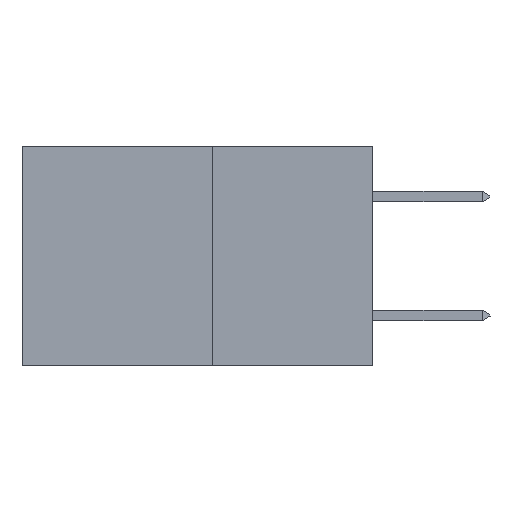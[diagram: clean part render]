
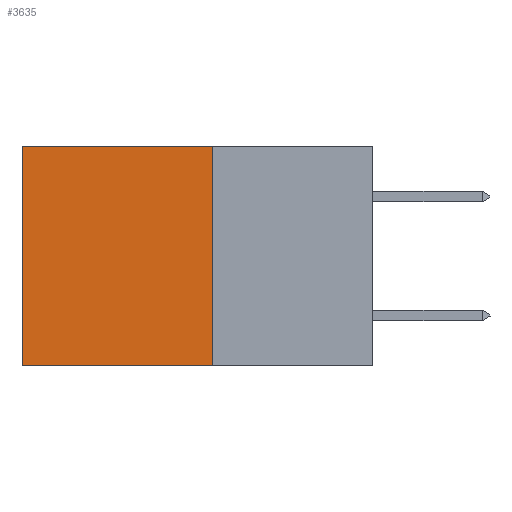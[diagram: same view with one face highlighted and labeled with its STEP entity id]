
A CAD part, left-side view. The second image highlights one B-rep face of the part: STEP entity #3635.
In plain terms, the highlighted planar face has unit normal (-1, 0, 0).
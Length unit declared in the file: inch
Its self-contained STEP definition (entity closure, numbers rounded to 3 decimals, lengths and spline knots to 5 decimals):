
#110 = VECTOR ( 'NONE', #1015, 39.37008 ) ;
#155 = CARTESIAN_POINT ( 'NONE',  ( 0.277, 0.27, -0.37 ) ) ;
#812 = CARTESIAN_POINT ( 'NONE',  ( 0.277, 0.59, -0.37 ) ) ;
#900 = ORIENTED_EDGE ( 'NONE', *, *, #6768, .F. ) ;
#988 = VECTOR ( 'NONE', #1818, 39.37008 ) ;
#1015 = DIRECTION ( 'NONE',  ( 0., 1., 0. ) ) ;
#1137 = DIRECTION ( 'NONE',  ( 1., 0., 0. ) ) ;
#1166 = DIRECTION ( 'NONE',  ( 0., 0., -1. ) ) ;
#1189 = PLANE ( 'NONE',  #7337 ) ;
#1203 = CARTESIAN_POINT ( 'NONE',  ( 0.277, 0.27, -0.37 ) ) ;
#1358 = EDGE_CURVE ( 'NONE', #4739, #5498, #2336, .T. ) ;
#1521 = EDGE_CURVE ( 'NONE', #5498, #5710, #2466, .T. ) ;
#1818 = DIRECTION ( 'NONE',  ( 0., 0., -1. ) ) ;
#1840 = DIRECTION ( 'NONE',  ( 0., 0., -1. ) ) ;
#1923 = ORIENTED_EDGE ( 'NONE', *, *, #1358, .T. ) ;
#2117 = FACE_OUTER_BOUND ( 'NONE', #4970, .T. ) ;
#2203 = VECTOR ( 'NONE', #1840, 39.37008 ) ;
#2336 = LINE ( 'NONE', #2471, #110 ) ;
#2352 = CARTESIAN_POINT ( 'NONE',  ( 0.277, 0.59, 0. ) ) ;
#2466 = LINE ( 'NONE', #812, #2203 ) ;
#2471 = CARTESIAN_POINT ( 'NONE',  ( 0.277, 0.27, 0. ) ) ;
#2958 = LINE ( 'NONE', #155, #988 ) ;
#3508 = VERTEX_POINT ( 'NONE', #5075 ) ;
#3635 = ADVANCED_FACE ( 'NONE', ( #2117 ), #1189, .F. ) ;
#3849 = DIRECTION ( 'NONE',  ( 0., 1., 0. ) ) ;
#4739 = VERTEX_POINT ( 'NONE', #9595 ) ;
#4970 = EDGE_LOOP ( 'NONE', ( #8831, #900, #5209, #1923 ) ) ;
#5075 = CARTESIAN_POINT ( 'NONE',  ( 0.277, 0.27, -0.37 ) ) ;
#5209 = ORIENTED_EDGE ( 'NONE', *, *, #7965, .F. ) ;
#5498 = VERTEX_POINT ( 'NONE', #2352 ) ;
#5710 = VERTEX_POINT ( 'NONE', #6478 ) ;
#6478 = CARTESIAN_POINT ( 'NONE',  ( 0.277, 0.59, -0.37 ) ) ;
#6768 = EDGE_CURVE ( 'NONE', #3508, #5710, #7169, .T. ) ;
#6955 = VECTOR ( 'NONE', #3849, 39.37008 ) ;
#7169 = LINE ( 'NONE', #9732, #6955 ) ;
#7337 = AXIS2_PLACEMENT_3D ( 'NONE', #1203, #1137, #1166 ) ;
#7965 = EDGE_CURVE ( 'NONE', #4739, #3508, #2958, .T. ) ;
#8831 = ORIENTED_EDGE ( 'NONE', *, *, #1521, .T. ) ;
#9595 = CARTESIAN_POINT ( 'NONE',  ( 0.277, 0.27, 0. ) ) ;
#9732 = CARTESIAN_POINT ( 'NONE',  ( 0.277, 0.27, -0.37 ) ) ;
